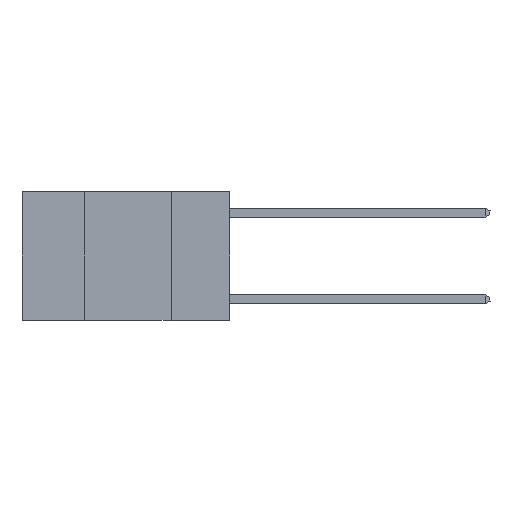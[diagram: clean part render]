
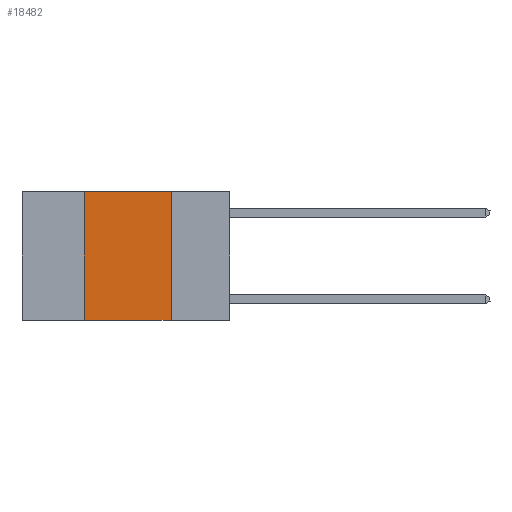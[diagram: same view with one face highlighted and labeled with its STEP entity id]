
A CAD part, left-side view. The second image highlights one B-rep face of the part: STEP entity #18482.
In plain terms, the highlighted planar face has unit normal (-1, 0, 0).
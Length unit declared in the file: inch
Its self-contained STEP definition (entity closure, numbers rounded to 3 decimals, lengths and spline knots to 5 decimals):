
#450 = VECTOR ( 'NONE', #26365, 39.37008 ) ;
#1983 = AXIS2_PLACEMENT_3D ( 'NONE', #24872, #7242, #22804 ) ;
#4162 = LINE ( 'NONE', #9000, #15376 ) ;
#5394 = EDGE_CURVE ( 'NONE', #19830, #19183, #4162, .T. ) ;
#6249 = VERTEX_POINT ( 'NONE', #12006 ) ;
#6562 = EDGE_CURVE ( 'NONE', #19183, #6249, #13241, .T. ) ;
#6916 = VECTOR ( 'NONE', #25583, 39.37008 ) ;
#7242 = DIRECTION ( 'NONE',  ( 1., 0., 0. ) ) ;
#8357 = CARTESIAN_POINT ( 'NONE',  ( 0., 0.17, -0.37 ) ) ;
#8695 = CARTESIAN_POINT ( 'NONE',  ( 0., 0.6, -0.37 ) ) ;
#9000 = CARTESIAN_POINT ( 'NONE',  ( 0., 0.42, 0. ) ) ;
#11106 = FACE_OUTER_BOUND ( 'NONE', #25271, .T. ) ;
#11248 = DIRECTION ( 'NONE',  ( 0., 0., 1. ) ) ;
#11652 = VERTEX_POINT ( 'NONE', #8357 ) ;
#12006 = CARTESIAN_POINT ( 'NONE',  ( 0., 0.17, 0. ) ) ;
#13241 = LINE ( 'NONE', #19504, #22954 ) ;
#13451 = ORIENTED_EDGE ( 'NONE', *, *, #5394, .F. ) ;
#13682 = PLANE ( 'NONE',  #1983 ) ;
#14331 = CARTESIAN_POINT ( 'NONE',  ( 0., 0.42, 0. ) ) ;
#15206 = DIRECTION ( 'NONE',  ( 0., -1., 0. ) ) ;
#15376 = VECTOR ( 'NONE', #11248, 39.37008 ) ;
#15514 = EDGE_CURVE ( 'NONE', #19830, #11652, #22776, .T. ) ;
#18231 = ORIENTED_EDGE ( 'NONE', *, *, #15514, .T. ) ;
#18482 = ADVANCED_FACE ( 'NONE', ( #11106 ), #13682, .F. ) ;
#18788 = LINE ( 'NONE', #21233, #6916 ) ;
#19183 = VERTEX_POINT ( 'NONE', #14331 ) ;
#19504 = CARTESIAN_POINT ( 'NONE',  ( 0., 0.6, 0. ) ) ;
#19830 = VERTEX_POINT ( 'NONE', #20732 ) ;
#20139 = ORIENTED_EDGE ( 'NONE', *, *, #6562, .F. ) ;
#20732 = CARTESIAN_POINT ( 'NONE',  ( 0., 0.42, -0.37 ) ) ;
#21233 = CARTESIAN_POINT ( 'NONE',  ( 0., 0.17, 0. ) ) ;
#21948 = ORIENTED_EDGE ( 'NONE', *, *, #25769, .F. ) ;
#22776 = LINE ( 'NONE', #8695, #450 ) ;
#22804 = DIRECTION ( 'NONE',  ( 0., 0., -1. ) ) ;
#22954 = VECTOR ( 'NONE', #15206, 39.37008 ) ;
#24872 = CARTESIAN_POINT ( 'NONE',  ( 0., 0.6, 0. ) ) ;
#25271 = EDGE_LOOP ( 'NONE', ( #21948, #20139, #13451, #18231 ) ) ;
#25583 = DIRECTION ( 'NONE',  ( 0., 0., -1. ) ) ;
#25769 = EDGE_CURVE ( 'NONE', #6249, #11652, #18788, .T. ) ;
#26365 = DIRECTION ( 'NONE',  ( 0., -1., 0. ) ) ;
